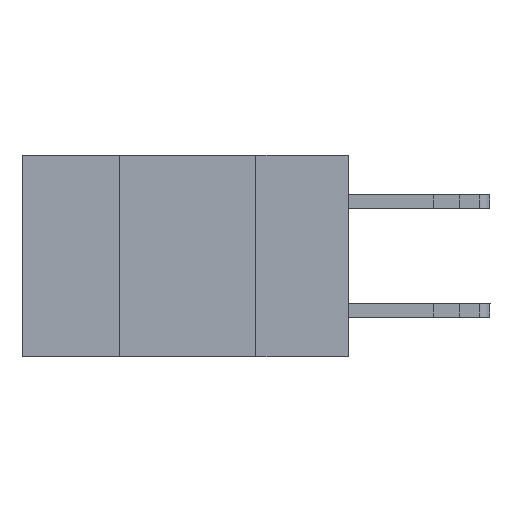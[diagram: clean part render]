
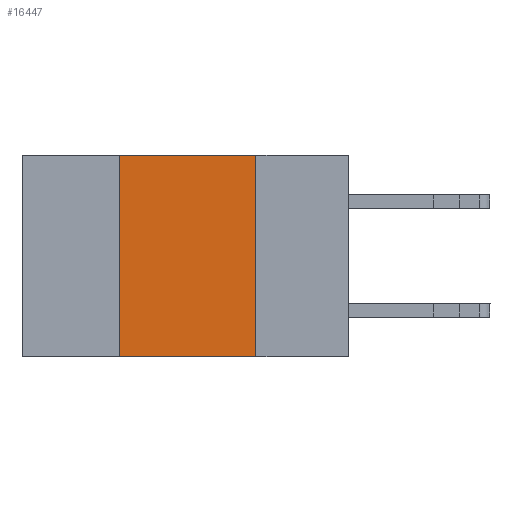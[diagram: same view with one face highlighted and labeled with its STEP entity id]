
A CAD part, left-side view. The second image highlights one B-rep face of the part: STEP entity #16447.
In plain terms, the highlighted planar face has unit normal (-1, 0, 0).
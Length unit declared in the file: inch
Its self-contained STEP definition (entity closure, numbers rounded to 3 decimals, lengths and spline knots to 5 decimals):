
#307 = VECTOR ( 'NONE', #15213, 39.37008 ) ;
#441 = AXIS2_PLACEMENT_3D ( 'NONE', #9031, #579, #10425 ) ;
#579 = DIRECTION ( 'NONE',  ( 1., 0., 0. ) ) ;
#588 = DIRECTION ( 'NONE',  ( 0., -1., 0. ) ) ;
#677 = CARTESIAN_POINT ( 'NONE',  ( 0., 0.6, 0. ) ) ;
#1590 = LINE ( 'NONE', #677, #16329 ) ;
#2508 = LINE ( 'NONE', #13080, #16754 ) ;
#2559 = EDGE_CURVE ( 'NONE', #17531, #7299, #1590, .T. ) ;
#4480 = EDGE_CURVE ( 'NONE', #16083, #16042, #4630, .T. ) ;
#4630 = LINE ( 'NONE', #17187, #11586 ) ;
#5257 = CARTESIAN_POINT ( 'NONE',  ( 0., 0.17, 0. ) ) ;
#5455 = CARTESIAN_POINT ( 'NONE',  ( 0., 0.42, -0.37 ) ) ;
#6984 = CARTESIAN_POINT ( 'NONE',  ( 0., 0.42, -0.37 ) ) ;
#7299 = VERTEX_POINT ( 'NONE', #5257 ) ;
#8610 = DIRECTION ( 'NONE',  ( 0., -1., 0. ) ) ;
#9031 = CARTESIAN_POINT ( 'NONE',  ( 0., 0.6, 0. ) ) ;
#9073 = ORIENTED_EDGE ( 'NONE', *, *, #2559, .F. ) ;
#9514 = CARTESIAN_POINT ( 'NONE',  ( 0., 0.17, -0.37 ) ) ;
#9961 = ORIENTED_EDGE ( 'NONE', *, *, #16774, .F. ) ;
#10137 = ORIENTED_EDGE ( 'NONE', *, *, #13164, .F. ) ;
#10425 = DIRECTION ( 'NONE',  ( 0., 0., -1. ) ) ;
#10561 = ORIENTED_EDGE ( 'NONE', *, *, #4480, .T. ) ;
#10665 = FACE_OUTER_BOUND ( 'NONE', #11068, .T. ) ;
#11068 = EDGE_LOOP ( 'NONE', ( #10137, #9073, #9961, #10561 ) ) ;
#11540 = LINE ( 'NONE', #6984, #307 ) ;
#11586 = VECTOR ( 'NONE', #8610, 39.37008 ) ;
#11971 = CARTESIAN_POINT ( 'NONE',  ( 0., 0.42, 0. ) ) ;
#13080 = CARTESIAN_POINT ( 'NONE',  ( 0., 0.17, -0.37 ) ) ;
#13164 = EDGE_CURVE ( 'NONE', #7299, #16042, #2508, .T. ) ;
#15213 = DIRECTION ( 'NONE',  ( 0., 0., 1. ) ) ;
#15833 = DIRECTION ( 'NONE',  ( 0., 0., -1. ) ) ;
#15874 = PLANE ( 'NONE',  #441 ) ;
#16042 = VERTEX_POINT ( 'NONE', #9514 ) ;
#16083 = VERTEX_POINT ( 'NONE', #5455 ) ;
#16329 = VECTOR ( 'NONE', #588, 39.37008 ) ;
#16447 = ADVANCED_FACE ( 'NONE', ( #10665 ), #15874, .F. ) ;
#16754 = VECTOR ( 'NONE', #15833, 39.37008 ) ;
#16774 = EDGE_CURVE ( 'NONE', #16083, #17531, #11540, .T. ) ;
#17187 = CARTESIAN_POINT ( 'NONE',  ( 0., 0.6, -0.37 ) ) ;
#17531 = VERTEX_POINT ( 'NONE', #11971 ) ;
